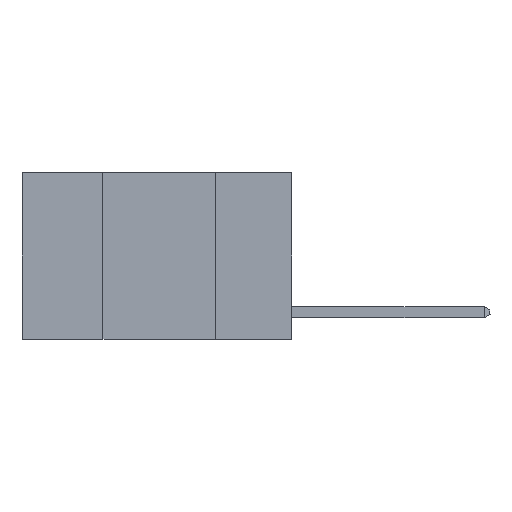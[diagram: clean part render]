
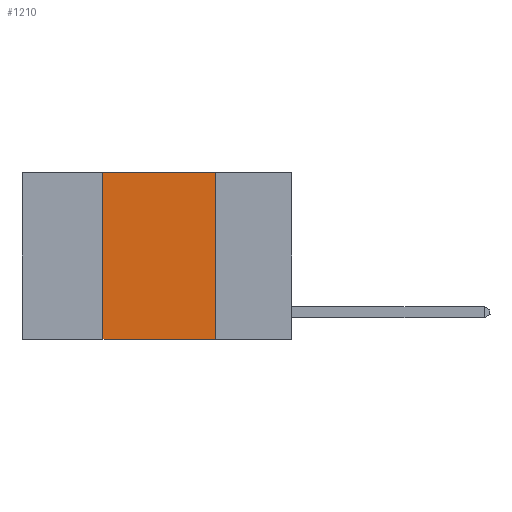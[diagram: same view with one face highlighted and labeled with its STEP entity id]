
A CAD part, left-side view. The second image highlights one B-rep face of the part: STEP entity #1210.
In plain terms, the highlighted planar face has unit normal (-1, 0, 0).
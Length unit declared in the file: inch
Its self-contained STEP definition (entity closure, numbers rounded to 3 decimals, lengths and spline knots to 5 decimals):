
#14 = CARTESIAN_POINT ( 'NONE',  ( 0., 0.42, 0. ) ) ;
#74 = VECTOR ( 'NONE', #11157, 39.37008 ) ;
#803 = VECTOR ( 'NONE', #2229, 39.37008 ) ;
#845 = ORIENTED_EDGE ( 'NONE', *, *, #11066, .F. ) ;
#1017 = CARTESIAN_POINT ( 'NONE',  ( 0., 0.6, 0. ) ) ;
#1210 = ADVANCED_FACE ( 'NONE', ( #6365 ), #2198, .F. ) ;
#1224 = DIRECTION ( 'NONE',  ( 1., 0., 0. ) ) ;
#1296 = VECTOR ( 'NONE', #11173, 39.37008 ) ;
#1621 = VERTEX_POINT ( 'NONE', #4280 ) ;
#1664 = EDGE_CURVE ( 'NONE', #8664, #1621, #11616, .T. ) ;
#2198 = PLANE ( 'NONE',  #9341 ) ;
#2229 = DIRECTION ( 'NONE',  ( 0., -1., 0. ) ) ;
#3087 = EDGE_LOOP ( 'NONE', ( #9692, #11816, #845, #11593 ) ) ;
#4280 = CARTESIAN_POINT ( 'NONE',  ( 0., 0.17, 0. ) ) ;
#4807 = CARTESIAN_POINT ( 'NONE',  ( 0., 0.6, -0.37 ) ) ;
#5025 = LINE ( 'NONE', #10028, #1296 ) ;
#5469 = CARTESIAN_POINT ( 'NONE',  ( 0., 0.42, -0.37 ) ) ;
#5479 = VERTEX_POINT ( 'NONE', #8545 ) ;
#5662 = CARTESIAN_POINT ( 'NONE',  ( 0., 0.17, 0. ) ) ;
#6365 = FACE_OUTER_BOUND ( 'NONE', #3087, .T. ) ;
#8545 = CARTESIAN_POINT ( 'NONE',  ( 0., 0.17, -0.37 ) ) ;
#8664 = VERTEX_POINT ( 'NONE', #14 ) ;
#8756 = LINE ( 'NONE', #5662, #10686 ) ;
#9123 = VERTEX_POINT ( 'NONE', #5469 ) ;
#9341 = AXIS2_PLACEMENT_3D ( 'NONE', #1017, #1224, #9382 ) ;
#9382 = DIRECTION ( 'NONE',  ( 0., 0., -1. ) ) ;
#9692 = ORIENTED_EDGE ( 'NONE', *, *, #13445, .F. ) ;
#10028 = CARTESIAN_POINT ( 'NONE',  ( 0., 0.42, 0. ) ) ;
#10207 = LINE ( 'NONE', #4807, #74 ) ;
#10686 = VECTOR ( 'NONE', #11936, 39.37008 ) ;
#11066 = EDGE_CURVE ( 'NONE', #9123, #8664, #5025, .T. ) ;
#11157 = DIRECTION ( 'NONE',  ( 0., -1., 0. ) ) ;
#11173 = DIRECTION ( 'NONE',  ( 0., 0., 1. ) ) ;
#11426 = EDGE_CURVE ( 'NONE', #9123, #5479, #10207, .T. ) ;
#11593 = ORIENTED_EDGE ( 'NONE', *, *, #11426, .T. ) ;
#11616 = LINE ( 'NONE', #11817, #803 ) ;
#11816 = ORIENTED_EDGE ( 'NONE', *, *, #1664, .F. ) ;
#11817 = CARTESIAN_POINT ( 'NONE',  ( 0., 0.6, 0. ) ) ;
#11936 = DIRECTION ( 'NONE',  ( 0., 0., -1. ) ) ;
#13445 = EDGE_CURVE ( 'NONE', #1621, #5479, #8756, .T. ) ;
